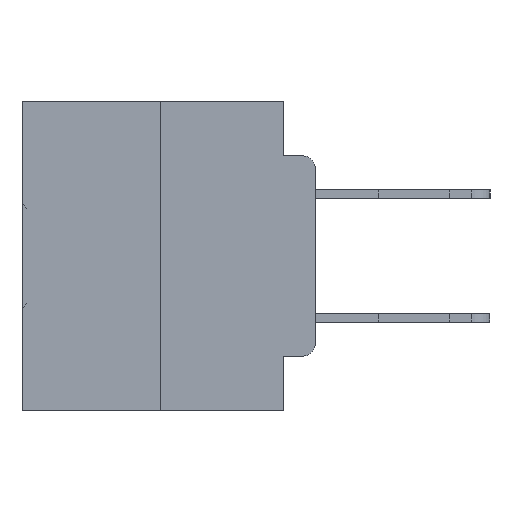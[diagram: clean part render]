
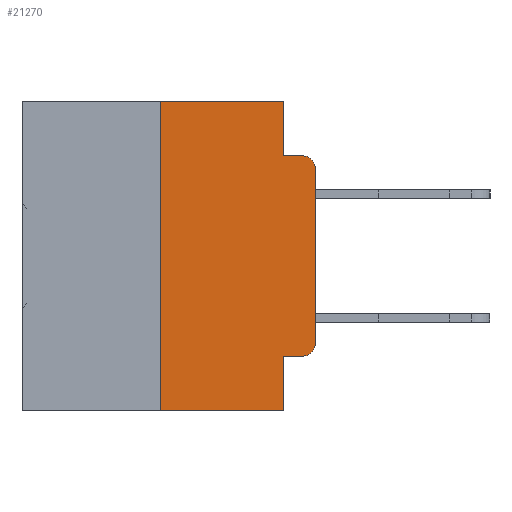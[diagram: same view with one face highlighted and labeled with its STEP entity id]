
A CAD part, left-side view. The second image highlights one B-rep face of the part: STEP entity #21270.
In plain terms, the highlighted planar face has unit normal (-1, 0, 0).
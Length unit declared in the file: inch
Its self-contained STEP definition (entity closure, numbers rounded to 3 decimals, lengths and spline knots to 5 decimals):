
#104 = CIRCLE ( 'NONE', #23721, 0.02 ) ;
#512 = LINE ( 'NONE', #5326, #28225 ) ;
#754 = LINE ( 'NONE', #2911, #35750 ) ;
#954 = DIRECTION ( 'NONE',  ( 0., 0., -1. ) ) ;
#1018 = ORIENTED_EDGE ( 'NONE', *, *, #35535, .T. ) ;
#1624 = DIRECTION ( 'NONE',  ( 0., -1., 0. ) ) ;
#2289 = EDGE_CURVE ( 'NONE', #18064, #23213, #12641, .T. ) ;
#2911 = CARTESIAN_POINT ( 'NONE',  ( 0., 0.051, 0. ) ) ;
#3140 = PLANE ( 'NONE',  #3226 ) ;
#3226 = AXIS2_PLACEMENT_3D ( 'NONE', #19731, #11551, #30798 ) ;
#4464 = VERTEX_POINT ( 'NONE', #6110 ) ;
#5037 = CARTESIAN_POINT ( 'NONE',  ( 0., 0.02, -0.4115 ) ) ;
#5326 = CARTESIAN_POINT ( 'NONE',  ( 0., 0.051, -0.0885 ) ) ;
#5900 = EDGE_CURVE ( 'NONE', #19159, #31381, #20573, .T. ) ;
#6110 = CARTESIAN_POINT ( 'NONE',  ( 0., 0.25, -0.5 ) ) ;
#6601 = EDGE_CURVE ( 'NONE', #13486, #31549, #18317, .T. ) ;
#8137 = DIRECTION ( 'NONE',  ( 0., -1., 0. ) ) ;
#8470 = EDGE_CURVE ( 'NONE', #33347, #8857, #104, .T. ) ;
#8857 = VERTEX_POINT ( 'NONE', #18709 ) ;
#8862 = ORIENTED_EDGE ( 'NONE', *, *, #28231, .F. ) ;
#8949 = CARTESIAN_POINT ( 'NONE',  ( 0., 0.25, 0. ) ) ;
#9557 = FACE_OUTER_BOUND ( 'NONE', #34825, .T. ) ;
#9594 = CARTESIAN_POINT ( 'NONE',  ( 0., 0.051, -0.4115 ) ) ;
#10795 = LINE ( 'NONE', #19918, #16379 ) ;
#10830 = LINE ( 'NONE', #15135, #24672 ) ;
#11464 = ORIENTED_EDGE ( 'NONE', *, *, #5900, .F. ) ;
#11551 = DIRECTION ( 'NONE',  ( 1., 0., 0. ) ) ;
#12579 = LINE ( 'NONE', #9594, #25539 ) ;
#12641 = LINE ( 'NONE', #29399, #33742 ) ;
#12860 = LINE ( 'NONE', #26459, #33965 ) ;
#13486 = VERTEX_POINT ( 'NONE', #13816 ) ;
#13816 = CARTESIAN_POINT ( 'NONE',  ( 0., 0., -0.1085 ) ) ;
#14673 = DIRECTION ( 'NONE',  ( -1., 0., 0. ) ) ;
#15135 = CARTESIAN_POINT ( 'NONE',  ( 0., 0., 0. ) ) ;
#15573 = ORIENTED_EDGE ( 'NONE', *, *, #8470, .T. ) ;
#15792 = VERTEX_POINT ( 'NONE', #24657 ) ;
#16190 = AXIS2_PLACEMENT_3D ( 'NONE', #31176, #14673, #33946 ) ;
#16379 = VECTOR ( 'NONE', #28247, 39.37008 ) ;
#17286 = ORIENTED_EDGE ( 'NONE', *, *, #21459, .T. ) ;
#17554 = DIRECTION ( 'NONE',  ( -1., 0., 0. ) ) ;
#17901 = DIRECTION ( 'NONE',  ( 0., 0., 1. ) ) ;
#18064 = VERTEX_POINT ( 'NONE', #8949 ) ;
#18317 = CIRCLE ( 'NONE', #16190, 0.02 ) ;
#18709 = CARTESIAN_POINT ( 'NONE',  ( 0., 0., -0.3915 ) ) ;
#19159 = VERTEX_POINT ( 'NONE', #22314 ) ;
#19576 = ORIENTED_EDGE ( 'NONE', *, *, #31330, .F. ) ;
#19731 = CARTESIAN_POINT ( 'NONE',  ( 0., 0.473, 0. ) ) ;
#19918 = CARTESIAN_POINT ( 'NONE',  ( 0., 0.25, 0. ) ) ;
#20573 = LINE ( 'NONE', #28095, #27041 ) ;
#21270 = ADVANCED_FACE ( 'NONE', ( #9557 ), #3140, .F. ) ;
#21459 = EDGE_CURVE ( 'NONE', #19159, #33347, #12579, .T. ) ;
#21461 = EDGE_CURVE ( 'NONE', #8857, #13486, #10830, .T. ) ;
#21968 = EDGE_CURVE ( 'NONE', #4464, #18064, #10795, .T. ) ;
#22314 = CARTESIAN_POINT ( 'NONE',  ( 0., 0.051, -0.4115 ) ) ;
#22659 = CARTESIAN_POINT ( 'NONE',  ( 0., 0.051, 0. ) ) ;
#23213 = VERTEX_POINT ( 'NONE', #22659 ) ;
#23721 = AXIS2_PLACEMENT_3D ( 'NONE', #34067, #17554, #954 ) ;
#24378 = ORIENTED_EDGE ( 'NONE', *, *, #21968, .F. ) ;
#24657 = CARTESIAN_POINT ( 'NONE',  ( 0., 0.051, -0.0885 ) ) ;
#24672 = VECTOR ( 'NONE', #17901, 39.37008 ) ;
#25366 = DIRECTION ( 'NONE',  ( 0., 0., -1. ) ) ;
#25539 = VECTOR ( 'NONE', #26153, 39.37008 ) ;
#26153 = DIRECTION ( 'NONE',  ( 0., -1., 0. ) ) ;
#26459 = CARTESIAN_POINT ( 'NONE',  ( 0., 0.473, -0.5 ) ) ;
#26670 = DIRECTION ( 'NONE',  ( 0., -1., 0. ) ) ;
#27041 = VECTOR ( 'NONE', #25366, 39.37008 ) ;
#27372 = ORIENTED_EDGE ( 'NONE', *, *, #6601, .T. ) ;
#28095 = CARTESIAN_POINT ( 'NONE',  ( 0., 0.051, 0. ) ) ;
#28225 = VECTOR ( 'NONE', #8137, 39.37008 ) ;
#28231 = EDGE_CURVE ( 'NONE', #23213, #15792, #754, .T. ) ;
#28247 = DIRECTION ( 'NONE',  ( 0., 0., 1. ) ) ;
#28382 = CARTESIAN_POINT ( 'NONE',  ( 0., 0.02, -0.0885 ) ) ;
#29399 = CARTESIAN_POINT ( 'NONE',  ( 0., 0.473, 0. ) ) ;
#30562 = DIRECTION ( 'NONE',  ( 0., 0., -1. ) ) ;
#30798 = DIRECTION ( 'NONE',  ( 0., 0., -1. ) ) ;
#31176 = CARTESIAN_POINT ( 'NONE',  ( 0., 0.02, -0.1085 ) ) ;
#31239 = ORIENTED_EDGE ( 'NONE', *, *, #2289, .F. ) ;
#31330 = EDGE_CURVE ( 'NONE', #15792, #31549, #512, .T. ) ;
#31381 = VERTEX_POINT ( 'NONE', #33079 ) ;
#31549 = VERTEX_POINT ( 'NONE', #28382 ) ;
#33079 = CARTESIAN_POINT ( 'NONE',  ( 0., 0.051, -0.5 ) ) ;
#33347 = VERTEX_POINT ( 'NONE', #5037 ) ;
#33742 = VECTOR ( 'NONE', #26670, 39.37008 ) ;
#33946 = DIRECTION ( 'NONE',  ( 0., 0., -1. ) ) ;
#33965 = VECTOR ( 'NONE', #1624, 39.37008 ) ;
#34067 = CARTESIAN_POINT ( 'NONE',  ( 0., 0.02, -0.3915 ) ) ;
#34692 = ORIENTED_EDGE ( 'NONE', *, *, #21461, .T. ) ;
#34825 = EDGE_LOOP ( 'NONE', ( #34692, #27372, #19576, #8862, #31239, #24378, #1018, #11464, #17286, #15573 ) ) ;
#35535 = EDGE_CURVE ( 'NONE', #4464, #31381, #12860, .T. ) ;
#35750 = VECTOR ( 'NONE', #30562, 39.37008 ) ;
